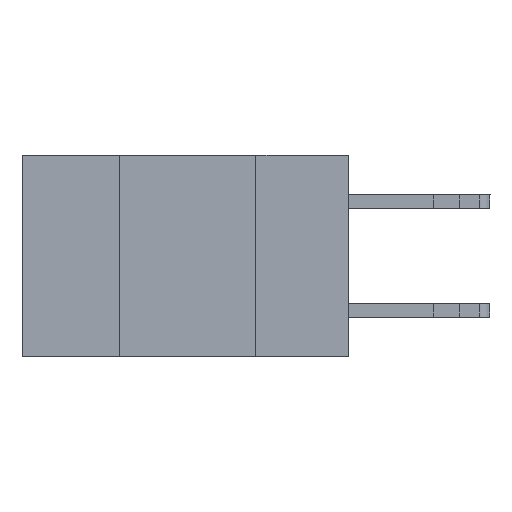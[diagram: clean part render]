
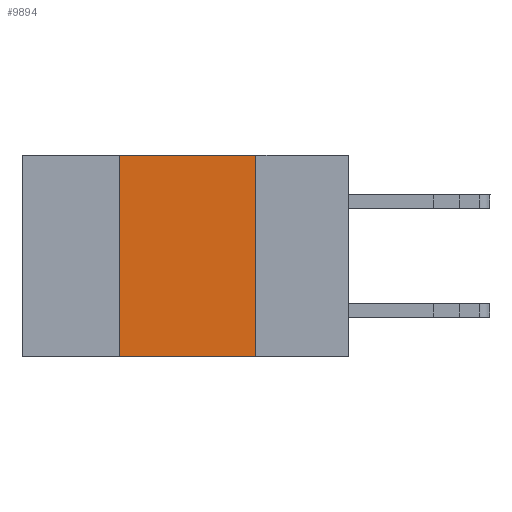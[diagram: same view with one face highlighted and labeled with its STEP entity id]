
A CAD part, left-side view. The second image highlights one B-rep face of the part: STEP entity #9894.
In plain terms, the highlighted planar face has unit normal (-1, 0, 0).
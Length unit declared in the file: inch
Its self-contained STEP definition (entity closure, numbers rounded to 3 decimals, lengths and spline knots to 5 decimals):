
#602 = LINE ( 'NONE', #13021, #8370 ) ;
#618 = CARTESIAN_POINT ( 'NONE',  ( 0., 0.6, 0. ) ) ;
#913 = VERTEX_POINT ( 'NONE', #6245 ) ;
#1430 = VERTEX_POINT ( 'NONE', #16306 ) ;
#2094 = EDGE_CURVE ( 'NONE', #913, #13029, #4486, .T. ) ;
#2148 = VECTOR ( 'NONE', #13429, 39.37008 ) ;
#2336 = DIRECTION ( 'NONE',  ( 0., 0., -1. ) ) ;
#3395 = DIRECTION ( 'NONE',  ( 0., 0., -1. ) ) ;
#4486 = LINE ( 'NONE', #9811, #9783 ) ;
#4516 = EDGE_CURVE ( 'NONE', #913, #1430, #12085, .T. ) ;
#5132 = CARTESIAN_POINT ( 'NONE',  ( 0., 0.17, 0. ) ) ;
#6245 = CARTESIAN_POINT ( 'NONE',  ( 0., 0.42, -0.37 ) ) ;
#7467 = PLANE ( 'NONE',  #12899 ) ;
#7615 = ORIENTED_EDGE ( 'NONE', *, *, #2094, .F. ) ;
#7780 = CARTESIAN_POINT ( 'NONE',  ( 0., 0.6, -0.37 ) ) ;
#8370 = VECTOR ( 'NONE', #3395, 39.37008 ) ;
#9166 = FACE_OUTER_BOUND ( 'NONE', #14125, .T. ) ;
#9450 = VERTEX_POINT ( 'NONE', #5132 ) ;
#9783 = VECTOR ( 'NONE', #9973, 39.37008 ) ;
#9811 = CARTESIAN_POINT ( 'NONE',  ( 0., 0.42, 0. ) ) ;
#9894 = ADVANCED_FACE ( 'NONE', ( #9166 ), #7467, .F. ) ;
#9973 = DIRECTION ( 'NONE',  ( 0., 0., 1. ) ) ;
#10058 = ORIENTED_EDGE ( 'NONE', *, *, #16845, .F. ) ;
#10296 = VECTOR ( 'NONE', #10766, 39.37008 ) ;
#10766 = DIRECTION ( 'NONE',  ( 0., -1., 0. ) ) ;
#11612 = EDGE_CURVE ( 'NONE', #9450, #1430, #602, .T. ) ;
#12085 = LINE ( 'NONE', #7780, #2148 ) ;
#12899 = AXIS2_PLACEMENT_3D ( 'NONE', #618, #14656, #2336 ) ;
#13021 = CARTESIAN_POINT ( 'NONE',  ( 0., 0.17, 0. ) ) ;
#13029 = VERTEX_POINT ( 'NONE', #17533 ) ;
#13429 = DIRECTION ( 'NONE',  ( 0., -1., 0. ) ) ;
#14125 = EDGE_LOOP ( 'NONE', ( #15684, #10058, #7615, #17475 ) ) ;
#14656 = DIRECTION ( 'NONE',  ( 1., 0., 0. ) ) ;
#15684 = ORIENTED_EDGE ( 'NONE', *, *, #11612, .F. ) ;
#16306 = CARTESIAN_POINT ( 'NONE',  ( 0., 0.17, -0.37 ) ) ;
#16359 = LINE ( 'NONE', #17620, #10296 ) ;
#16845 = EDGE_CURVE ( 'NONE', #13029, #9450, #16359, .T. ) ;
#17475 = ORIENTED_EDGE ( 'NONE', *, *, #4516, .T. ) ;
#17533 = CARTESIAN_POINT ( 'NONE',  ( 0., 0.42, 0. ) ) ;
#17620 = CARTESIAN_POINT ( 'NONE',  ( 0., 0.6, 0. ) ) ;
